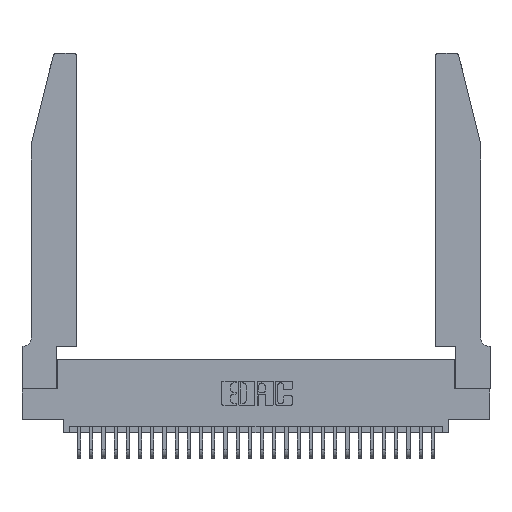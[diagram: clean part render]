
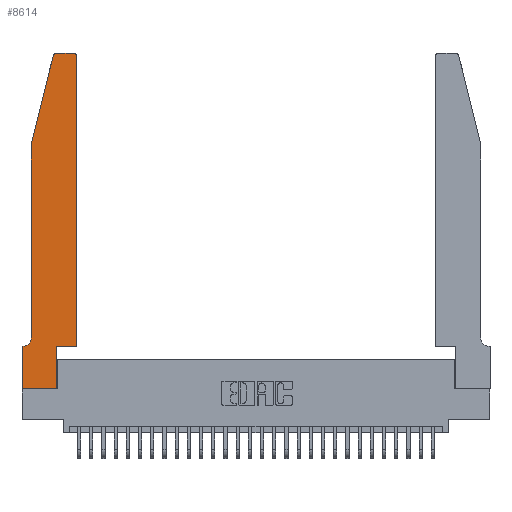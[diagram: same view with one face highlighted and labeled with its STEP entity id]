
A CAD part, top view. The second image highlights one B-rep face of the part: STEP entity #8614.
In plain terms, the highlighted planar face has unit normal (0, 0, 1).
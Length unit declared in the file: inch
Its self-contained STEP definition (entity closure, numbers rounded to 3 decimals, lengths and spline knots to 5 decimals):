
#59 = LINE ( 'NONE', #6748, #6639 ) ;
#87 = CARTESIAN_POINT ( 'NONE',  ( 0.2605, 2.75, 0.37 ) ) ;
#159 = VECTOR ( 'NONE', #25507, 39.37008 ) ;
#167 = CARTESIAN_POINT ( 'NONE',  ( 0., 0., 0.37 ) ) ;
#332 = CIRCLE ( 'NONE', #16409, 0.07 ) ;
#1086 = ORIENTED_EDGE ( 'NONE', *, *, #28447, .T. ) ;
#1792 = VECTOR ( 'NONE', #13039, 39.37008 ) ;
#1932 = VERTEX_POINT ( 'NONE', #10124 ) ;
#2221 = EDGE_CURVE ( 'NONE', #6006, #6034, #332, .T. ) ;
#2716 = CARTESIAN_POINT ( 'NONE',  ( 0.4205, 2.72, 0.37 ) ) ;
#2996 = VERTEX_POINT ( 'NONE', #24396 ) ;
#3180 = CARTESIAN_POINT ( 'NONE',  ( 0.2865, 0.35, 0.37 ) ) ;
#3684 = DIRECTION ( 'NONE',  ( 0., -1., 0. ) ) ;
#3718 = LINE ( 'NONE', #3180, #9493 ) ;
#4738 = CARTESIAN_POINT ( 'NONE',  ( 0.0055, 0.35, 0.37 ) ) ;
#5120 = CARTESIAN_POINT ( 'NONE',  ( 0.4505, 0.35, 0.37 ) ) ;
#5183 = DIRECTION ( 'NONE',  ( 1., 0., 0. ) ) ;
#5357 = ORIENTED_EDGE ( 'NONE', *, *, #2221, .T. ) ;
#5553 = VERTEX_POINT ( 'NONE', #19835 ) ;
#5643 = DIRECTION ( 'NONE',  ( 0., 1., 0. ) ) ;
#5825 = EDGE_CURVE ( 'NONE', #5553, #6006, #17869, .T. ) ;
#6006 = VERTEX_POINT ( 'NONE', #24248 ) ;
#6034 = VERTEX_POINT ( 'NONE', #4738 ) ;
#6639 = VECTOR ( 'NONE', #7613, 39.37008 ) ;
#6748 = CARTESIAN_POINT ( 'NONE',  ( 0.0755, 0.35, 0.37 ) ) ;
#6752 = DIRECTION ( 'NONE',  ( 0., 0., 1. ) ) ;
#6849 = DIRECTION ( 'NONE',  ( 0., 0., -1. ) ) ;
#6874 = ORIENTED_EDGE ( 'NONE', *, *, #18017, .T. ) ;
#6879 = DIRECTION ( 'NONE',  ( 0., 1., 0. ) ) ;
#7613 = DIRECTION ( 'NONE',  ( -1., 0., 0. ) ) ;
#8194 = EDGE_CURVE ( 'NONE', #13745, #10831, #31306, .T. ) ;
#8357 = LINE ( 'NONE', #10608, #1792 ) ;
#8368 = CARTESIAN_POINT ( 'NONE',  ( 0., 0., 0.37 ) ) ;
#8428 = ORIENTED_EDGE ( 'NONE', *, *, #9728, .T. ) ;
#8614 = ADVANCED_FACE ( 'NONE', ( #20707 ), #21495, .T. ) ;
#9493 = VECTOR ( 'NONE', #5643, 39.37008 ) ;
#9728 = EDGE_CURVE ( 'NONE', #1932, #15814, #3718, .T. ) ;
#10124 = CARTESIAN_POINT ( 'NONE',  ( 0.2865, 0., 0.37 ) ) ;
#10350 = ORIENTED_EDGE ( 'NONE', *, *, #13110, .T. ) ;
#10608 = CARTESIAN_POINT ( 'NONE',  ( 0., 0., 0.37 ) ) ;
#10831 = VERTEX_POINT ( 'NONE', #19065 ) ;
#11189 = VECTOR ( 'NONE', #16416, 39.37008 ) ;
#11565 = CARTESIAN_POINT ( 'NONE',  ( 0.0755, 2., 0.37 ) ) ;
#11567 = VERTEX_POINT ( 'NONE', #17838 ) ;
#11743 = EDGE_CURVE ( 'NONE', #2996, #11567, #13566, .T. ) ;
#12821 = AXIS2_PLACEMENT_3D ( 'NONE', #14016, #31055, #16530 ) ;
#12973 = AXIS2_PLACEMENT_3D ( 'NONE', #14048, #6752, #23911 ) ;
#13039 = DIRECTION ( 'NONE',  ( 0., -1., 0. ) ) ;
#13110 = EDGE_CURVE ( 'NONE', #11567, #5553, #30626, .T. ) ;
#13566 = CIRCLE ( 'NONE', #12821, 0.03 ) ;
#13745 = VERTEX_POINT ( 'NONE', #28304 ) ;
#14016 = CARTESIAN_POINT ( 'NONE',  ( 0.284, 2.72, 0.37 ) ) ;
#14048 = CARTESIAN_POINT ( 'NONE',  ( 0., 0.35, 0.37 ) ) ;
#14468 = EDGE_CURVE ( 'NONE', #6034, #15882, #59, .T. ) ;
#15148 = VERTEX_POINT ( 'NONE', #5120 ) ;
#15331 = ORIENTED_EDGE ( 'NONE', *, *, #24857, .T. ) ;
#15729 = LINE ( 'NONE', #87, #21491 ) ;
#15814 = VERTEX_POINT ( 'NONE', #20132 ) ;
#15838 = EDGE_LOOP ( 'NONE', ( #15331, #22619, #10350, #17674, #5357, #25671, #6874, #1086, #8428, #27956, #23006, #23765 ) ) ;
#15882 = VERTEX_POINT ( 'NONE', #24314 ) ;
#16409 = AXIS2_PLACEMENT_3D ( 'NONE', #21588, #6849, #24008 ) ;
#16416 = DIRECTION ( 'NONE',  ( -0.239, -0.971, 0. ) ) ;
#16530 = DIRECTION ( 'NONE',  ( 1., 0., 0. ) ) ;
#16975 = CARTESIAN_POINT ( 'NONE',  ( 0.4505, 0.35, 0.37 ) ) ;
#17674 = ORIENTED_EDGE ( 'NONE', *, *, #5825, .T. ) ;
#17736 = EDGE_CURVE ( 'NONE', #15814, #15148, #18397, .T. ) ;
#17838 = CARTESIAN_POINT ( 'NONE',  ( 0.25487, 2.72718, 0.37 ) ) ;
#17869 = LINE ( 'NONE', #25857, #24336 ) ;
#18017 = EDGE_CURVE ( 'NONE', #15882, #28242, #8357, .T. ) ;
#18397 = LINE ( 'NONE', #16975, #22580 ) ;
#19065 = CARTESIAN_POINT ( 'NONE',  ( 0.4205, 2.75, 0.37 ) ) ;
#19833 = DIRECTION ( 'NONE',  ( -1., 0., 0. ) ) ;
#19835 = CARTESIAN_POINT ( 'NONE',  ( 0.0755, 2., 0.37 ) ) ;
#19922 = DIRECTION ( 'NONE',  ( 0., 0., 1. ) ) ;
#20132 = CARTESIAN_POINT ( 'NONE',  ( 0.2865, 0.35, 0.37 ) ) ;
#20707 = FACE_OUTER_BOUND ( 'NONE', #15838, .T. ) ;
#21491 = VECTOR ( 'NONE', #19833, 39.37008 ) ;
#21495 = PLANE ( 'NONE',  #12973 ) ;
#21588 = CARTESIAN_POINT ( 'NONE',  ( 0.0055, 0.42, 0.37 ) ) ;
#21994 = DIRECTION ( 'NONE',  ( 1., 0., 0. ) ) ;
#22571 = VECTOR ( 'NONE', #6879, 39.37008 ) ;
#22580 = VECTOR ( 'NONE', #21994, 39.37008 ) ;
#22619 = ORIENTED_EDGE ( 'NONE', *, *, #11743, .T. ) ;
#23006 = ORIENTED_EDGE ( 'NONE', *, *, #27185, .T. ) ;
#23765 = ORIENTED_EDGE ( 'NONE', *, *, #8194, .T. ) ;
#23911 = DIRECTION ( 'NONE',  ( 1., 0., 0. ) ) ;
#24008 = DIRECTION ( 'NONE',  ( -1., 0., 0. ) ) ;
#24040 = CARTESIAN_POINT ( 'NONE',  ( 0.4505, 0.35, 0.37 ) ) ;
#24248 = CARTESIAN_POINT ( 'NONE',  ( 0.0755, 0.42, 0.37 ) ) ;
#24314 = CARTESIAN_POINT ( 'NONE',  ( 0., 0.35, 0.37 ) ) ;
#24336 = VECTOR ( 'NONE', #3684, 39.37008 ) ;
#24396 = CARTESIAN_POINT ( 'NONE',  ( 0.284, 2.75, 0.37 ) ) ;
#24857 = EDGE_CURVE ( 'NONE', #10831, #2996, #15729, .T. ) ;
#25507 = DIRECTION ( 'NONE',  ( 1., 0., 0. ) ) ;
#25671 = ORIENTED_EDGE ( 'NONE', *, *, #14468, .T. ) ;
#25857 = CARTESIAN_POINT ( 'NONE',  ( 0.0755, 2., 0.37 ) ) ;
#27185 = EDGE_CURVE ( 'NONE', #15148, #13745, #28269, .T. ) ;
#27956 = ORIENTED_EDGE ( 'NONE', *, *, #17736, .T. ) ;
#28242 = VERTEX_POINT ( 'NONE', #167 ) ;
#28269 = LINE ( 'NONE', #24040, #22571 ) ;
#28304 = CARTESIAN_POINT ( 'NONE',  ( 0.4505, 2.72, 0.37 ) ) ;
#28447 = EDGE_CURVE ( 'NONE', #28242, #1932, #31178, .T. ) ;
#28951 = AXIS2_PLACEMENT_3D ( 'NONE', #2716, #19922, #5183 ) ;
#30626 = LINE ( 'NONE', #11565, #11189 ) ;
#31055 = DIRECTION ( 'NONE',  ( 0., 0., 1. ) ) ;
#31178 = LINE ( 'NONE', #8368, #159 ) ;
#31306 = CIRCLE ( 'NONE', #28951, 0.03 ) ;
